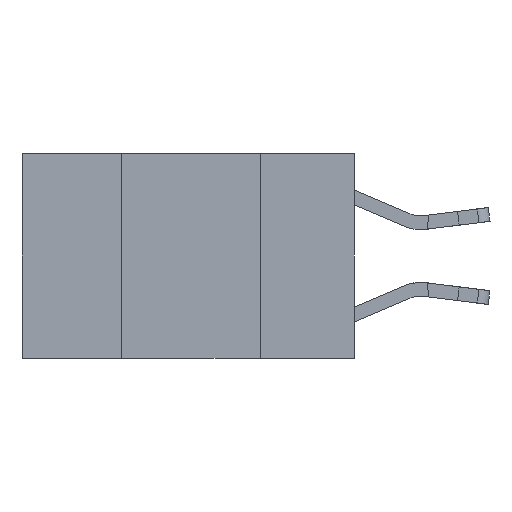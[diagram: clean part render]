
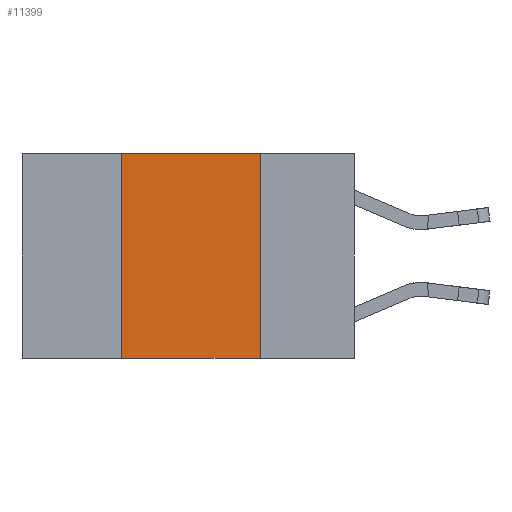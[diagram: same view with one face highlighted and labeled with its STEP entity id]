
A CAD part, left-side view. The second image highlights one B-rep face of the part: STEP entity #11399.
In plain terms, the highlighted planar face has unit normal (-1, 0, 0).
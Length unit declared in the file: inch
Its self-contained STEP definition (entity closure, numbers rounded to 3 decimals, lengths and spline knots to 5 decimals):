
#932 = CARTESIAN_POINT ( 'NONE',  ( 0., 0.42, -0.37 ) ) ;
#1072 = CARTESIAN_POINT ( 'NONE',  ( 0., 0.17, 0. ) ) ;
#1109 = ORIENTED_EDGE ( 'NONE', *, *, #8300, .F. ) ;
#1229 = DIRECTION ( 'NONE',  ( 0., -1., 0. ) ) ;
#1510 = DIRECTION ( 'NONE',  ( 0., 0., 1. ) ) ;
#1576 = DIRECTION ( 'NONE',  ( 0., 0., -1. ) ) ;
#2149 = VECTOR ( 'NONE', #1229, 39.37008 ) ;
#2563 = DIRECTION ( 'NONE',  ( 0., 0., -1. ) ) ;
#3713 = LINE ( 'NONE', #7359, #8092 ) ;
#4541 = CARTESIAN_POINT ( 'NONE',  ( 0., 0.17, -0.37 ) ) ;
#4562 = VECTOR ( 'NONE', #1510, 39.37008 ) ;
#4694 = VECTOR ( 'NONE', #2563, 39.37008 ) ;
#5019 = CARTESIAN_POINT ( 'NONE',  ( 0., 0.17, 0. ) ) ;
#5125 = VERTEX_POINT ( 'NONE', #5019 ) ;
#5582 = LINE ( 'NONE', #9726, #4562 ) ;
#5834 = CARTESIAN_POINT ( 'NONE',  ( 0., 0.6, 0. ) ) ;
#6707 = CARTESIAN_POINT ( 'NONE',  ( 0., 0.6, -0.37 ) ) ;
#6793 = LINE ( 'NONE', #6707, #2149 ) ;
#7359 = CARTESIAN_POINT ( 'NONE',  ( 0., 0.6, 0. ) ) ;
#7662 = VERTEX_POINT ( 'NONE', #932 ) ;
#7969 = LINE ( 'NONE', #1072, #4694 ) ;
#8092 = VECTOR ( 'NONE', #12906, 39.37008 ) ;
#8300 = EDGE_CURVE ( 'NONE', #7662, #15302, #5582, .T. ) ;
#9402 = ORIENTED_EDGE ( 'NONE', *, *, #15479, .T. ) ;
#9624 = FACE_OUTER_BOUND ( 'NONE', #17251, .T. ) ;
#9726 = CARTESIAN_POINT ( 'NONE',  ( 0., 0.42, 0. ) ) ;
#9730 = ORIENTED_EDGE ( 'NONE', *, *, #13717, .F. ) ;
#10277 = ORIENTED_EDGE ( 'NONE', *, *, #13531, .F. ) ;
#10950 = PLANE ( 'NONE',  #14217 ) ;
#11399 = ADVANCED_FACE ( 'NONE', ( #9624 ), #10950, .F. ) ;
#11592 = VERTEX_POINT ( 'NONE', #4541 ) ;
#12357 = DIRECTION ( 'NONE',  ( 1., 0., 0. ) ) ;
#12906 = DIRECTION ( 'NONE',  ( 0., -1., 0. ) ) ;
#13531 = EDGE_CURVE ( 'NONE', #15302, #5125, #3713, .T. ) ;
#13717 = EDGE_CURVE ( 'NONE', #5125, #11592, #7969, .T. ) ;
#14217 = AXIS2_PLACEMENT_3D ( 'NONE', #5834, #12357, #1576 ) ;
#14286 = CARTESIAN_POINT ( 'NONE',  ( 0., 0.42, 0. ) ) ;
#15302 = VERTEX_POINT ( 'NONE', #14286 ) ;
#15479 = EDGE_CURVE ( 'NONE', #7662, #11592, #6793, .T. ) ;
#17251 = EDGE_LOOP ( 'NONE', ( #9730, #10277, #1109, #9402 ) ) ;
